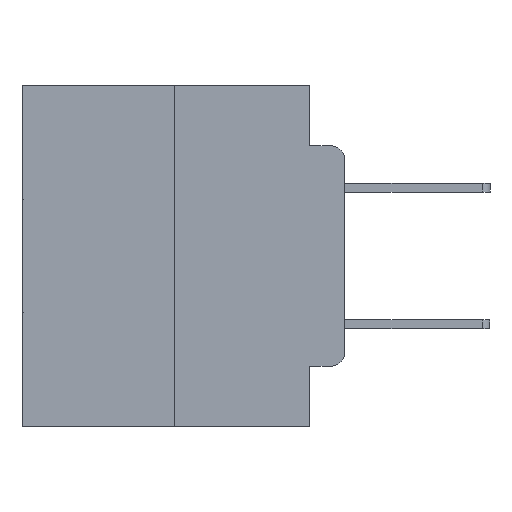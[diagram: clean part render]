
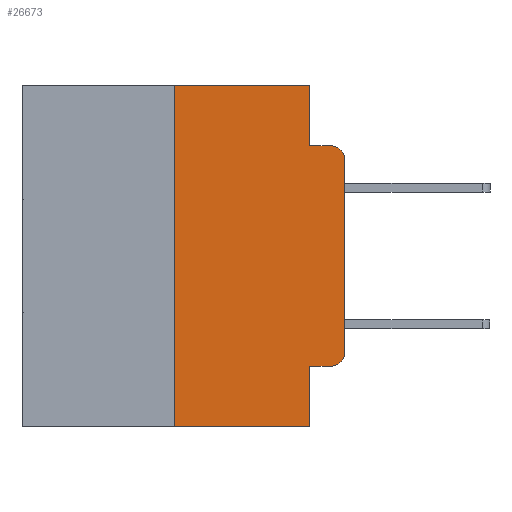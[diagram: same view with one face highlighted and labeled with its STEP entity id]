
A CAD part, left-side view. The second image highlights one B-rep face of the part: STEP entity #26673.
In plain terms, the highlighted planar face has unit normal (-1, 0, 0).
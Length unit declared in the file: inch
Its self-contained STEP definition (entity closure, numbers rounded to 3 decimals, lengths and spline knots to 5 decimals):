
#72 = LINE ( 'NONE', #9457, #22143 ) ;
#396 = CARTESIAN_POINT ( 'NONE',  ( 0., 0.051, 0. ) ) ;
#520 = ORIENTED_EDGE ( 'NONE', *, *, #9443, .T. ) ;
#688 = EDGE_CURVE ( 'NONE', #22165, #16280, #7819, .T. ) ;
#1018 = LINE ( 'NONE', #12491, #22992 ) ;
#1040 = EDGE_CURVE ( 'NONE', #22165, #22664, #10468, .T. ) ;
#1118 = ORIENTED_EDGE ( 'NONE', *, *, #2148, .F. ) ;
#1242 = DIRECTION ( 'NONE',  ( -1., 0., 0. ) ) ;
#1268 = CARTESIAN_POINT ( 'NONE',  ( 0., 0.02, -0.4115 ) ) ;
#1554 = VERTEX_POINT ( 'NONE', #11765 ) ;
#2148 = EDGE_CURVE ( 'NONE', #22664, #25700, #7064, .T. ) ;
#2832 = DIRECTION ( 'NONE',  ( 0., -1., 0. ) ) ;
#3903 = DIRECTION ( 'NONE',  ( 0., 0., -1. ) ) ;
#4306 = CARTESIAN_POINT ( 'NONE',  ( 0., 0.02, -0.3915 ) ) ;
#4433 = EDGE_CURVE ( 'NONE', #24493, #15086, #22246, .T. ) ;
#4714 = VECTOR ( 'NONE', #24735, 39.37008 ) ;
#5142 = AXIS2_PLACEMENT_3D ( 'NONE', #25375, #6543, #21336 ) ;
#5501 = CARTESIAN_POINT ( 'NONE',  ( 0., 0.051, -0.5 ) ) ;
#6140 = CIRCLE ( 'NONE', #17922, 0.02 ) ;
#6150 = ORIENTED_EDGE ( 'NONE', *, *, #4433, .T. ) ;
#6416 = CARTESIAN_POINT ( 'NONE',  ( 0., 0.051, -0.4115 ) ) ;
#6519 = DIRECTION ( 'NONE',  ( 0., 0., -1. ) ) ;
#6543 = DIRECTION ( 'NONE',  ( 1., 0., 0. ) ) ;
#6881 = AXIS2_PLACEMENT_3D ( 'NONE', #14153, #1242, #16292 ) ;
#6898 = CIRCLE ( 'NONE', #6881, 0.02 ) ;
#6900 = ORIENTED_EDGE ( 'NONE', *, *, #9153, .T. ) ;
#7064 = LINE ( 'NONE', #26928, #23850 ) ;
#7069 = EDGE_CURVE ( 'NONE', #24493, #16280, #72, .T. ) ;
#7194 = CARTESIAN_POINT ( 'NONE',  ( 0., 0.051, -0.4115 ) ) ;
#7548 = ORIENTED_EDGE ( 'NONE', *, *, #1040, .F. ) ;
#7564 = CARTESIAN_POINT ( 'NONE',  ( 0., 0.25, 0. ) ) ;
#7819 = LINE ( 'NONE', #10337, #12161 ) ;
#8338 = VECTOR ( 'NONE', #2832, 39.37008 ) ;
#9153 = EDGE_CURVE ( 'NONE', #15086, #23885, #6140, .T. ) ;
#9417 = CARTESIAN_POINT ( 'NONE',  ( 0., 0., -0.1085 ) ) ;
#9443 = EDGE_CURVE ( 'NONE', #23885, #14040, #22016, .T. ) ;
#9457 = CARTESIAN_POINT ( 'NONE',  ( 0., 0.051, 0. ) ) ;
#9923 = EDGE_LOOP ( 'NONE', ( #520, #19467, #21182, #14471, #1118, #7548, #11647, #16585, #6150, #6900 ) ) ;
#10160 = VECTOR ( 'NONE', #20108, 39.37008 ) ;
#10337 = CARTESIAN_POINT ( 'NONE',  ( 0., 0.473, -0.5 ) ) ;
#10464 = CARTESIAN_POINT ( 'NONE',  ( 0., 0.25, 0. ) ) ;
#10468 = LINE ( 'NONE', #10464, #4714 ) ;
#11647 = ORIENTED_EDGE ( 'NONE', *, *, #688, .T. ) ;
#11765 = CARTESIAN_POINT ( 'NONE',  ( 0., 0.02, -0.0885 ) ) ;
#12161 = VECTOR ( 'NONE', #18160, 39.37008 ) ;
#12491 = CARTESIAN_POINT ( 'NONE',  ( 0., 0.051, 0. ) ) ;
#12928 = VERTEX_POINT ( 'NONE', #16462 ) ;
#14040 = VERTEX_POINT ( 'NONE', #9417 ) ;
#14153 = CARTESIAN_POINT ( 'NONE',  ( 0., 0.02, -0.1085 ) ) ;
#14291 = CARTESIAN_POINT ( 'NONE',  ( 0., 0.25, -0.5 ) ) ;
#14471 = ORIENTED_EDGE ( 'NONE', *, *, #27177, .F. ) ;
#14674 = LINE ( 'NONE', #17810, #8338 ) ;
#14736 = DIRECTION ( 'NONE',  ( 0., -1., 0. ) ) ;
#15086 = VERTEX_POINT ( 'NONE', #1268 ) ;
#16280 = VERTEX_POINT ( 'NONE', #5501 ) ;
#16292 = DIRECTION ( 'NONE',  ( 0., 0., -1. ) ) ;
#16462 = CARTESIAN_POINT ( 'NONE',  ( 0., 0.051, -0.0885 ) ) ;
#16585 = ORIENTED_EDGE ( 'NONE', *, *, #7069, .F. ) ;
#17227 = DIRECTION ( 'NONE',  ( 0., -1., 0. ) ) ;
#17810 = CARTESIAN_POINT ( 'NONE',  ( 0., 0.051, -0.0885 ) ) ;
#17922 = AXIS2_PLACEMENT_3D ( 'NONE', #4306, #19239, #6519 ) ;
#18007 = CARTESIAN_POINT ( 'NONE',  ( 0., 0., -0.3915 ) ) ;
#18051 = CARTESIAN_POINT ( 'NONE',  ( 0., 0., 0. ) ) ;
#18160 = DIRECTION ( 'NONE',  ( 0., -1., 0. ) ) ;
#19239 = DIRECTION ( 'NONE',  ( -1., 0., 0. ) ) ;
#19259 = PLANE ( 'NONE',  #5142 ) ;
#19467 = ORIENTED_EDGE ( 'NONE', *, *, #20444, .T. ) ;
#19479 = FACE_OUTER_BOUND ( 'NONE', #9923, .T. ) ;
#20108 = DIRECTION ( 'NONE',  ( 0., 0., 1. ) ) ;
#20444 = EDGE_CURVE ( 'NONE', #14040, #1554, #6898, .T. ) ;
#21182 = ORIENTED_EDGE ( 'NONE', *, *, #23844, .F. ) ;
#21336 = DIRECTION ( 'NONE',  ( 0., 0., -1. ) ) ;
#21600 = VECTOR ( 'NONE', #17227, 39.37008 ) ;
#22016 = LINE ( 'NONE', #18051, #10160 ) ;
#22143 = VECTOR ( 'NONE', #25472, 39.37008 ) ;
#22165 = VERTEX_POINT ( 'NONE', #14291 ) ;
#22246 = LINE ( 'NONE', #6416, #21600 ) ;
#22664 = VERTEX_POINT ( 'NONE', #7564 ) ;
#22992 = VECTOR ( 'NONE', #3903, 39.37008 ) ;
#23844 = EDGE_CURVE ( 'NONE', #12928, #1554, #14674, .T. ) ;
#23850 = VECTOR ( 'NONE', #14736, 39.37008 ) ;
#23885 = VERTEX_POINT ( 'NONE', #18007 ) ;
#24493 = VERTEX_POINT ( 'NONE', #7194 ) ;
#24735 = DIRECTION ( 'NONE',  ( 0., 0., 1. ) ) ;
#25375 = CARTESIAN_POINT ( 'NONE',  ( 0., 0.473, 0. ) ) ;
#25472 = DIRECTION ( 'NONE',  ( 0., 0., -1. ) ) ;
#25700 = VERTEX_POINT ( 'NONE', #396 ) ;
#26673 = ADVANCED_FACE ( 'NONE', ( #19479 ), #19259, .F. ) ;
#26928 = CARTESIAN_POINT ( 'NONE',  ( 0., 0.473, 0. ) ) ;
#27177 = EDGE_CURVE ( 'NONE', #25700, #12928, #1018, .T. ) ;
